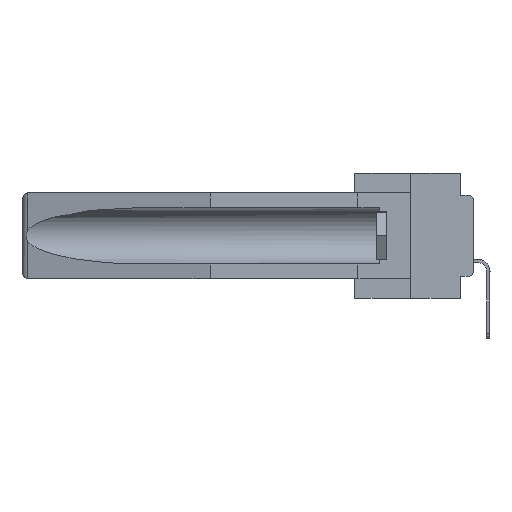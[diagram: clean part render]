
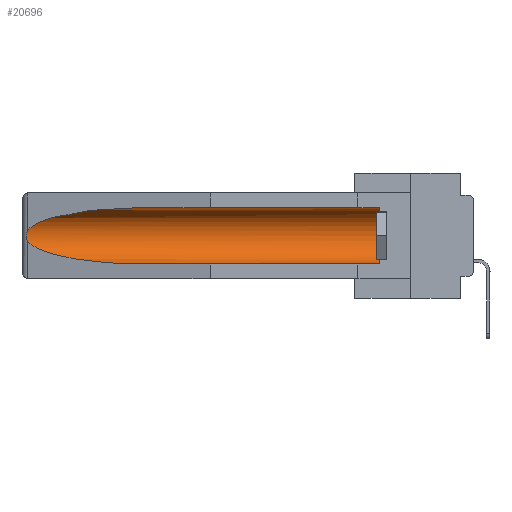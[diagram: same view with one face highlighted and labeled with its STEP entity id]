
A CAD part, left-side view. The second image highlights one B-rep face of the part: STEP entity #20696.
In plain terms, the highlighted cylindrical face has radius 2.857 mm (diameter 5.715 mm), a partial arc.
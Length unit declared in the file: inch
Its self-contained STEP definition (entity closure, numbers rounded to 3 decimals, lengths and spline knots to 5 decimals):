
#62 = CARTESIAN_POINT ( 'NONE',  ( 0.155, 1.07973, -0.059 ) ) ;
#324 = ORIENTED_EDGE ( 'NONE', *, *, #3119, .T. ) ;
#624 = VECTOR ( 'NONE', #26260, 39.37008 ) ;
#831 = CARTESIAN_POINT ( 'NONE',  ( 0.26597, 1.5296, -0.19026 ) ) ;
#1815 = VERTEX_POINT ( 'NONE', #15827 ) ;
#2737 = CARTESIAN_POINT ( 'NONE',  ( 0.155, -0.30754, -0.284 ) ) ;
#3000 = EDGE_LOOP ( 'NONE', ( #22104, #4215, #8067, #23371, #324, #14291 ) ) ;
#3119 = EDGE_CURVE ( 'NONE', #31675, #19566, #13761, .T. ) ;
#3252 = LINE ( 'NONE', #2737, #624 ) ;
#3401 = CARTESIAN_POINT ( 'NONE',  ( 0.2673, 1.5327, -0.16383 ) ) ;
#3748 = CARTESIAN_POINT ( 'NONE',  ( 0.2675, 1.53308, -0.16763 ) ) ;
#4215 = ORIENTED_EDGE ( 'NONE', *, *, #27045, .T. ) ;
#5278 = CARTESIAN_POINT ( 'NONE',  ( 0.155, 0.126, -0.1715 ) ) ;
#5847 = CARTESIAN_POINT ( 'NONE',  ( 0.155, 0.126, -0.284 ) ) ;
#5888 = EDGE_CURVE ( 'NONE', #18370, #24948, #10721, .T. ) ;
#6036 = CARTESIAN_POINT ( 'NONE',  ( 0.155, 0.126, -0.059 ) ) ;
#6186 = CARTESIAN_POINT ( 'NONE',  ( 0.26537, 1.52718, -0.19328 ) ) ;
#6360 = CARTESIAN_POINT ( 'NONE',  ( 0.2673, 1.53269, -0.17917 ) ) ;
#6695 = CARTESIAN_POINT ( 'NONE',  ( 0.26597, 1.52961, -0.15275 ) ) ;
#6987 = CARTESIAN_POINT ( 'NONE',  ( 0.155, 1.07973, -0.284 ) ) ;
#7788 = DIRECTION ( 'NONE',  ( 0., 1., 0. ) ) ;
#8067 = ORIENTED_EDGE ( 'NONE', *, *, #5888, .T. ) ;
#10222 = CARTESIAN_POINT ( 'NONE',  ( 0.155, -0.30754, -0.1715 ) ) ;
#10654 = EDGE_CURVE ( 'NONE', #31675, #24948, #3252, .T. ) ;
#10721 =( BOUNDED_CURVE ( )  B_SPLINE_CURVE ( 3, ( #23029, #25279, #19922, #6987 ),
 .UNSPECIFIED., .F., .F. ) 
 B_SPLINE_CURVE_WITH_KNOTS ( ( 4, 4 ),
 ( 0.1948, 1.5708 ),
 .UNSPECIFIED. ) 
 CURVE ( )  GEOMETRIC_REPRESENTATION_ITEM ( )  RATIONAL_B_SPLINE_CURVE ( ( 1., 0.848, 0.848, 1. ) ) 
 REPRESENTATION_ITEM ( '' )  );
#13662 = FACE_OUTER_BOUND ( 'NONE', #3000, .T. ) ;
#13761 = CIRCLE ( 'NONE', #28648, 0.1125 ) ;
#13972 = CARTESIAN_POINT ( 'NONE',  ( 0.2675, 1.53308, -0.17534 ) ) ;
#14291 = ORIENTED_EDGE ( 'NONE', *, *, #21934, .T. ) ;
#14925 = AXIS2_PLACEMENT_3D ( 'NONE', #10222, #7788, #26777 ) ;
#15827 = CARTESIAN_POINT ( 'NONE',  ( 0.26537, 1.52718, -0.14972 ) ) ;
#17127 = EDGE_CURVE ( 'NONE', #22694, #1815, #34104, .T. ) ;
#18370 = VERTEX_POINT ( 'NONE', #25658 ) ;
#19343 = CARTESIAN_POINT ( 'NONE',  ( 0.25451, 1.48313, -0.09465 ) ) ;
#19485 = CARTESIAN_POINT ( 'NONE',  ( 0.26537, 1.52718, -0.14972 ) ) ;
#19566 = VERTEX_POINT ( 'NONE', #6036 ) ;
#19922 = CARTESIAN_POINT ( 'NONE',  ( 0.21114, 1.30732, -0.284 ) ) ;
#20696 = ADVANCED_FACE ( 'NONE', ( #13662 ), #21068, .F. ) ;
#21068 = CYLINDRICAL_SURFACE ( 'NONE', #14925, 0.1125 ) ;
#21226 = DIRECTION ( 'NONE',  ( 0., 1., 0. ) ) ;
#21558 = LINE ( 'NONE', #29184, #27021 ) ;
#21934 = EDGE_CURVE ( 'NONE', #19566, #22694, #21558, .T. ) ;
#22104 = ORIENTED_EDGE ( 'NONE', *, *, #17127, .T. ) ;
#22694 = VERTEX_POINT ( 'NONE', #62 ) ;
#23029 = CARTESIAN_POINT ( 'NONE',  ( 0.26537, 1.52718, -0.19328 ) ) ;
#23371 = ORIENTED_EDGE ( 'NONE', *, *, #10654, .F. ) ;
#23651 = CARTESIAN_POINT ( 'NONE',  ( 0.155, 1.07973, -0.284 ) ) ;
#23667 = CARTESIAN_POINT ( 'NONE',  ( 0.155, 1.07973, -0.059 ) ) ;
#23757 = DIRECTION ( 'NONE',  ( 0., -1., 0. ) ) ;
#24488 = CARTESIAN_POINT ( 'NONE',  ( 0.26655, 1.53094, -0.18657 ) ) ;
#24948 = VERTEX_POINT ( 'NONE', #23651 ) ;
#25279 = CARTESIAN_POINT ( 'NONE',  ( 0.25451, 1.48313, -0.24835 ) ) ;
#25658 = CARTESIAN_POINT ( 'NONE',  ( 0.26537, 1.52718, -0.19328 ) ) ;
#26260 = DIRECTION ( 'NONE',  ( 0., 1., 0. ) ) ;
#26777 = DIRECTION ( 'NONE',  ( 0., 0., 1. ) ) ;
#26780 = CARTESIAN_POINT ( 'NONE',  ( 0.26537, 1.52718, -0.14972 ) ) ;
#27021 = VECTOR ( 'NONE', #21226, 39.37008 ) ;
#27045 = EDGE_CURVE ( 'NONE', #1815, #18370, #30636, .T. ) ;
#27086 = CARTESIAN_POINT ( 'NONE',  ( 0.26654, 1.53092, -0.15636 ) ) ;
#28648 = AXIS2_PLACEMENT_3D ( 'NONE', #5278, #23757, #28959 ) ;
#28959 = DIRECTION ( 'NONE',  ( 0., 0., 1. ) ) ;
#29184 = CARTESIAN_POINT ( 'NONE',  ( 0.155, -0.30754, -0.059 ) ) ;
#30636 = B_SPLINE_CURVE_WITH_KNOTS ( 'NONE', 3,
 ( #19485, #6695, #27086, #3401, #3748, #13972, #6360, #24488, #831, #6186 ),
 .UNSPECIFIED., .F., .F.,
 ( 4, 2, 2, 2, 4 ),
 ( 0., 0.00029, 0.00058, 0.00087, 0.00117 ),
 .UNSPECIFIED. ) ;
#31633 = CARTESIAN_POINT ( 'NONE',  ( 0.21114, 1.30732, -0.059 ) ) ;
#31675 = VERTEX_POINT ( 'NONE', #5847 ) ;
#34104 =( BOUNDED_CURVE ( )  B_SPLINE_CURVE ( 3, ( #23667, #31633, #19343, #26780 ),
 .UNSPECIFIED., .F., .F. ) 
 B_SPLINE_CURVE_WITH_KNOTS ( ( 4, 4 ),
 ( 4.71239, 6.08839 ),
 .UNSPECIFIED. ) 
 CURVE ( )  GEOMETRIC_REPRESENTATION_ITEM ( )  RATIONAL_B_SPLINE_CURVE ( ( 1., 0.848, 0.848, 1. ) ) 
 REPRESENTATION_ITEM ( '' )  );
